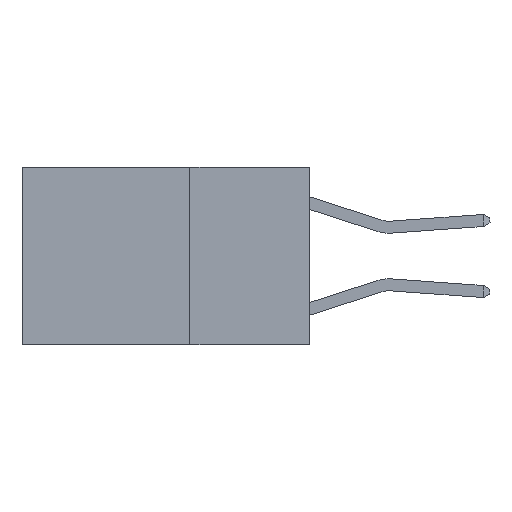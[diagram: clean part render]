
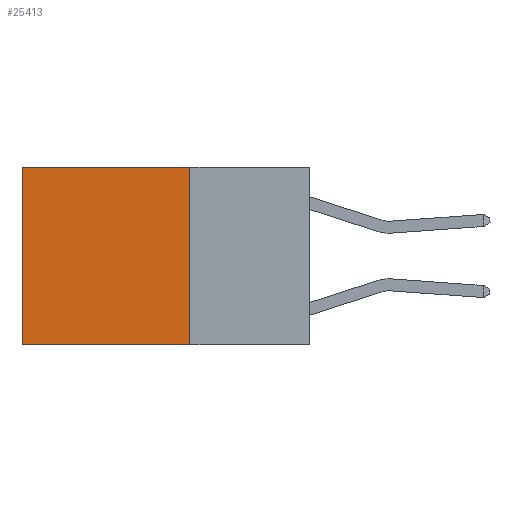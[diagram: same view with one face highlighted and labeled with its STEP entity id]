
A CAD part, left-side view. The second image highlights one B-rep face of the part: STEP entity #25413.
In plain terms, the highlighted planar face has unit normal (-1, 0, 0).
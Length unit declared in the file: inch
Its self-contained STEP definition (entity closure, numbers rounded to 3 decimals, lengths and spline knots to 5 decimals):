
#91 = LINE ( 'NONE', #1604, #13175 ) ;
#523 = DIRECTION ( 'NONE',  ( 0., 0., -1. ) ) ;
#747 = CARTESIAN_POINT ( 'NONE',  ( 0.2625, 0.25, 0. ) ) ;
#1604 = CARTESIAN_POINT ( 'NONE',  ( 0.2625, 0.25, 0. ) ) ;
#1828 = DIRECTION ( 'NONE',  ( 0., 0., -1. ) ) ;
#3568 = ORIENTED_EDGE ( 'NONE', *, *, #5090, .F. ) ;
#4501 = ORIENTED_EDGE ( 'NONE', *, *, #5788, .T. ) ;
#4669 = CARTESIAN_POINT ( 'NONE',  ( 0.2625, 0.6, 0. ) ) ;
#4796 = EDGE_CURVE ( 'NONE', #6918, #17000, #91, .T. ) ;
#5070 = DIRECTION ( 'NONE',  ( 0., 0., -1. ) ) ;
#5090 = EDGE_CURVE ( 'NONE', #6918, #10540, #11126, .T. ) ;
#5113 = LINE ( 'NONE', #4669, #22816 ) ;
#5567 = CARTESIAN_POINT ( 'NONE',  ( 0.2625, 0.25, -0.37 ) ) ;
#5788 = EDGE_CURVE ( 'NONE', #17000, #17409, #5113, .T. ) ;
#6248 = PLANE ( 'NONE',  #11624 ) ;
#6918 = VERTEX_POINT ( 'NONE', #9052 ) ;
#7130 = VECTOR ( 'NONE', #5070, 39.37008 ) ;
#9052 = CARTESIAN_POINT ( 'NONE',  ( 0.2625, 0.25, 0. ) ) ;
#10540 = VERTEX_POINT ( 'NONE', #14285 ) ;
#11126 = LINE ( 'NONE', #747, #7130 ) ;
#11489 = LINE ( 'NONE', #5567, #14183 ) ;
#11624 = AXIS2_PLACEMENT_3D ( 'NONE', #12501, #14656, #1828 ) ;
#12501 = CARTESIAN_POINT ( 'NONE',  ( 0.2625, 0.25, 0. ) ) ;
#12795 = CARTESIAN_POINT ( 'NONE',  ( 0.2625, 0.6, 0. ) ) ;
#13175 = VECTOR ( 'NONE', #25427, 39.37008 ) ;
#14183 = VECTOR ( 'NONE', #14452, 39.37008 ) ;
#14285 = CARTESIAN_POINT ( 'NONE',  ( 0.2625, 0.25, -0.37 ) ) ;
#14452 = DIRECTION ( 'NONE',  ( 0., 1., 0. ) ) ;
#14656 = DIRECTION ( 'NONE',  ( 1., 0., 0. ) ) ;
#15836 = ORIENTED_EDGE ( 'NONE', *, *, #23859, .F. ) ;
#17000 = VERTEX_POINT ( 'NONE', #12795 ) ;
#17409 = VERTEX_POINT ( 'NONE', #24975 ) ;
#19842 = EDGE_LOOP ( 'NONE', ( #4501, #15836, #3568, #21210 ) ) ;
#21210 = ORIENTED_EDGE ( 'NONE', *, *, #4796, .T. ) ;
#22816 = VECTOR ( 'NONE', #523, 39.37008 ) ;
#23859 = EDGE_CURVE ( 'NONE', #10540, #17409, #11489, .T. ) ;
#24975 = CARTESIAN_POINT ( 'NONE',  ( 0.2625, 0.6, -0.37 ) ) ;
#25413 = ADVANCED_FACE ( 'NONE', ( #26272 ), #6248, .F. ) ;
#25427 = DIRECTION ( 'NONE',  ( 0., 1., 0. ) ) ;
#26272 = FACE_OUTER_BOUND ( 'NONE', #19842, .T. ) ;
